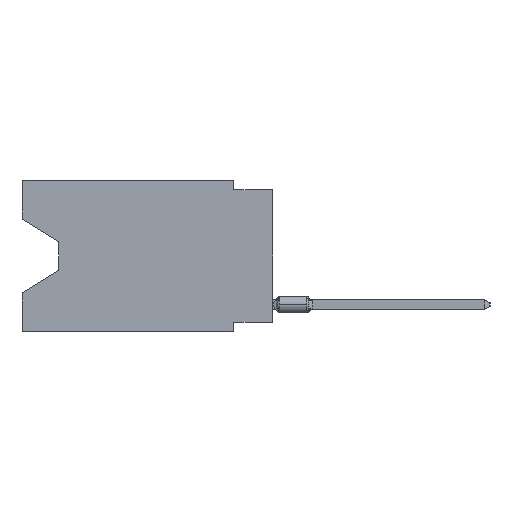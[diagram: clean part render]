
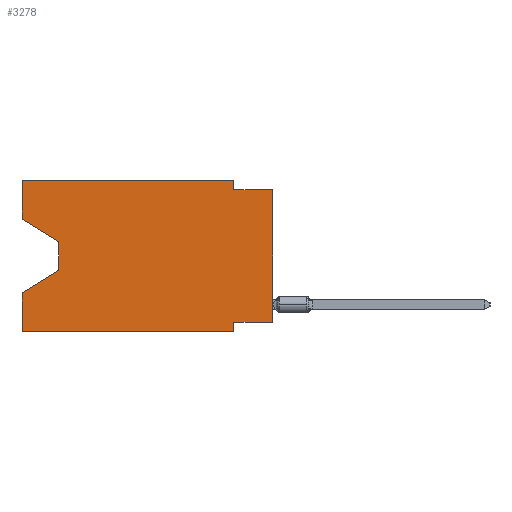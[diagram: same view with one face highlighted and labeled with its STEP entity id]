
A CAD part, left-side view. The second image highlights one B-rep face of the part: STEP entity #3278.
In plain terms, the highlighted planar face has unit normal (-1, 0, 0).
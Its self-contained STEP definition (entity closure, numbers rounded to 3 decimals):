
#803 = PLANE ( 'NONE',  #50660 ) ;
#1333 = VECTOR ( 'NONE', #57784, 1000. ) ;
#1486 = DIRECTION ( 'NONE',  ( 1., 0., 0. ) ) ;
#2002 = CARTESIAN_POINT ( 'NONE',  ( 0., 16.383, -7.36 ) ) ;
#2130 = CARTESIAN_POINT ( 'NONE',  ( 0., 2.54, 0. ) ) ;
#3278 = ADVANCED_FACE ( 'NONE', ( #32874 ), #803, .F. ) ;
#3888 = DIRECTION ( 'NONE',  ( 0., -0.855, -0.519 ) ) ;
#4047 = VECTOR ( 'NONE', #60823, 1000. ) ;
#4169 = VERTEX_POINT ( 'NONE', #23880 ) ;
#4537 = CARTESIAN_POINT ( 'NONE',  ( 0., 2.54, -9.906 ) ) ;
#5286 = ORIENTED_EDGE ( 'NONE', *, *, #61017, .T. ) ;
#5486 = CARTESIAN_POINT ( 'NONE',  ( 0., 2.54, -0.635 ) ) ;
#6067 = CARTESIAN_POINT ( 'NONE',  ( 0., 13.97, -4.013 ) ) ;
#6266 = CARTESIAN_POINT ( 'NONE',  ( 0., 2.54, -9.906 ) ) ;
#7118 = ORIENTED_EDGE ( 'NONE', *, *, #36547, .F. ) ;
#7205 = EDGE_CURVE ( 'NONE', #37999, #31700, #62146, .T. ) ;
#8161 = VERTEX_POINT ( 'NONE', #38242 ) ;
#8513 = LINE ( 'NONE', #14087, #4047 ) ;
#13145 = EDGE_CURVE ( 'NONE', #32600, #31700, #46646, .T. ) ;
#14087 = CARTESIAN_POINT ( 'NONE',  ( 0., 0., -9.271 ) ) ;
#14448 = CARTESIAN_POINT ( 'NONE',  ( 0., 2.54, 0. ) ) ;
#15188 = DIRECTION ( 'NONE',  ( 0., 0., 1. ) ) ;
#15367 = CARTESIAN_POINT ( 'NONE',  ( 0., 0., 0. ) ) ;
#16338 = VECTOR ( 'NONE', #41568, 1000. ) ;
#16516 = ORIENTED_EDGE ( 'NONE', *, *, #56605, .F. ) ;
#18087 = LINE ( 'NONE', #6266, #47087 ) ;
#18544 = DIRECTION ( 'NONE',  ( 0., -1., 0. ) ) ;
#18770 = CARTESIAN_POINT ( 'NONE',  ( 0., 16.383, -9.906 ) ) ;
#19230 = CARTESIAN_POINT ( 'NONE',  ( 0., 16.383, 0. ) ) ;
#19255 = VECTOR ( 'NONE', #55803, 1000. ) ;
#20482 = CARTESIAN_POINT ( 'NONE',  ( 0., 13.97, -5.893 ) ) ;
#20973 = CARTESIAN_POINT ( 'NONE',  ( 0., 13.97, -5.893 ) ) ;
#23880 = CARTESIAN_POINT ( 'NONE',  ( 0., 0., -9.271 ) ) ;
#23975 = VECTOR ( 'NONE', #53356, 1000. ) ;
#24260 = DIRECTION ( 'NONE',  ( 0., 0., -1. ) ) ;
#24857 = EDGE_LOOP ( 'NONE', ( #66274, #5286, #49618, #48967, #55232, #35533, #64570, #43968, #16516, #34166, #32055, #7118 ) ) ;
#24979 = LINE ( 'NONE', #57047, #51802 ) ;
#26293 = CARTESIAN_POINT ( 'NONE',  ( 0., 0., -0.635 ) ) ;
#26960 = CARTESIAN_POINT ( 'NONE',  ( 0., 16.383, 0. ) ) ;
#27914 = VERTEX_POINT ( 'NONE', #26293 ) ;
#29143 = CARTESIAN_POINT ( 'NONE',  ( 0., 13.97, -4.013 ) ) ;
#29836 = LINE ( 'NONE', #29143, #31159 ) ;
#31159 = VECTOR ( 'NONE', #24260, 1000. ) ;
#31700 = VERTEX_POINT ( 'NONE', #2002 ) ;
#32055 = ORIENTED_EDGE ( 'NONE', *, *, #53510, .F. ) ;
#32600 = VERTEX_POINT ( 'NONE', #20973 ) ;
#32874 = FACE_OUTER_BOUND ( 'NONE', #24857, .T. ) ;
#33217 = DIRECTION ( 'NONE',  ( 0., 0., -1. ) ) ;
#33534 = LINE ( 'NONE', #54432, #19255 ) ;
#33813 = EDGE_CURVE ( 'NONE', #63724, #62451, #66781, .T. ) ;
#34031 = EDGE_CURVE ( 'NONE', #37999, #56810, #60769, .T. ) ;
#34166 = ORIENTED_EDGE ( 'NONE', *, *, #33813, .F. ) ;
#34246 = LINE ( 'NONE', #15367, #23975 ) ;
#35533 = ORIENTED_EDGE ( 'NONE', *, *, #64192, .F. ) ;
#36547 = EDGE_CURVE ( 'NONE', #8161, #42294, #24979, .T. ) ;
#36951 = EDGE_CURVE ( 'NONE', #4169, #27914, #34246, .T. ) ;
#37999 = VERTEX_POINT ( 'NONE', #18770 ) ;
#38242 = CARTESIAN_POINT ( 'NONE',  ( 0., 16.383, -2.546 ) ) ;
#38832 = CARTESIAN_POINT ( 'NONE',  ( 0., 16.383, -9.906 ) ) ;
#39196 = VECTOR ( 'NONE', #18544, 1000. ) ;
#41033 = EDGE_CURVE ( 'NONE', #8161, #60072, #46441, .T. ) ;
#41568 = DIRECTION ( 'NONE',  ( 0., 0., 1. ) ) ;
#42294 = VERTEX_POINT ( 'NONE', #49490 ) ;
#43968 = ORIENTED_EDGE ( 'NONE', *, *, #36951, .T. ) ;
#46441 = LINE ( 'NONE', #51669, #52225 ) ;
#46646 = LINE ( 'NONE', #20482, #1333 ) ;
#47087 = VECTOR ( 'NONE', #60617, 1000. ) ;
#48170 = EDGE_CURVE ( 'NONE', #4169, #66154, #8513, .T. ) ;
#48661 = CARTESIAN_POINT ( 'NONE',  ( 0., 2.54, -9.271 ) ) ;
#48967 = ORIENTED_EDGE ( 'NONE', *, *, #7205, .F. ) ;
#49490 = CARTESIAN_POINT ( 'NONE',  ( 0., 16.383, 0. ) ) ;
#49618 = ORIENTED_EDGE ( 'NONE', *, *, #13145, .T. ) ;
#50660 = AXIS2_PLACEMENT_3D ( 'NONE', #26960, #1486, #33217 ) ;
#51081 = VECTOR ( 'NONE', #60081, 1000. ) ;
#51669 = CARTESIAN_POINT ( 'NONE',  ( 0., 16.383, -2.546 ) ) ;
#51802 = VECTOR ( 'NONE', #15188, 1000. ) ;
#52225 = VECTOR ( 'NONE', #3888, 1000. ) ;
#53356 = DIRECTION ( 'NONE',  ( 0., 0., 1. ) ) ;
#53510 = EDGE_CURVE ( 'NONE', #42294, #63724, #66329, .T. ) ;
#54432 = CARTESIAN_POINT ( 'NONE',  ( 0., 0., -0.635 ) ) ;
#55232 = ORIENTED_EDGE ( 'NONE', *, *, #34031, .T. ) ;
#55803 = DIRECTION ( 'NONE',  ( 0., -1., 0. ) ) ;
#56314 = DIRECTION ( 'NONE',  ( 0., 0., -1. ) ) ;
#56605 = EDGE_CURVE ( 'NONE', #62451, #27914, #33534, .T. ) ;
#56810 = VERTEX_POINT ( 'NONE', #4537 ) ;
#57047 = CARTESIAN_POINT ( 'NONE',  ( 0., 16.383, 0. ) ) ;
#57784 = DIRECTION ( 'NONE',  ( 0., 0.855, -0.519 ) ) ;
#60072 = VERTEX_POINT ( 'NONE', #6067 ) ;
#60081 = DIRECTION ( 'NONE',  ( 0., -1., 0. ) ) ;
#60617 = DIRECTION ( 'NONE',  ( 0., 0., -1. ) ) ;
#60769 = LINE ( 'NONE', #38832, #51081 ) ;
#60823 = DIRECTION ( 'NONE',  ( 0., 1., 0. ) ) ;
#61017 = EDGE_CURVE ( 'NONE', #60072, #32600, #29836, .T. ) ;
#62146 = LINE ( 'NONE', #68411, #16338 ) ;
#62451 = VERTEX_POINT ( 'NONE', #5486 ) ;
#63724 = VERTEX_POINT ( 'NONE', #2130 ) ;
#64192 = EDGE_CURVE ( 'NONE', #66154, #56810, #18087, .T. ) ;
#64570 = ORIENTED_EDGE ( 'NONE', *, *, #48170, .F. ) ;
#66154 = VERTEX_POINT ( 'NONE', #48661 ) ;
#66274 = ORIENTED_EDGE ( 'NONE', *, *, #41033, .T. ) ;
#66329 = LINE ( 'NONE', #19230, #39196 ) ;
#66606 = VECTOR ( 'NONE', #56314, 1000. ) ;
#66781 = LINE ( 'NONE', #14448, #66606 ) ;
#68411 = CARTESIAN_POINT ( 'NONE',  ( 0., 16.383, 0. ) ) ;
